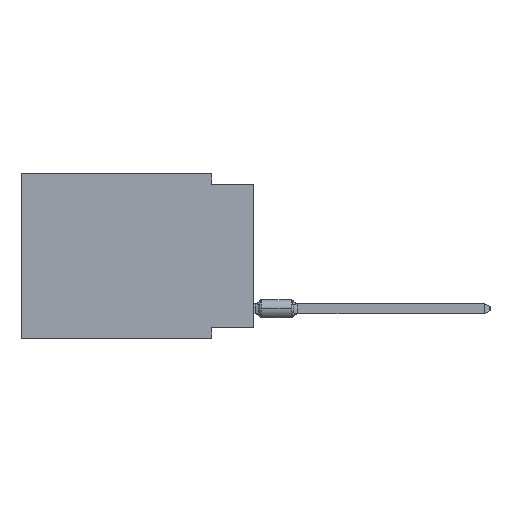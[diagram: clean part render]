
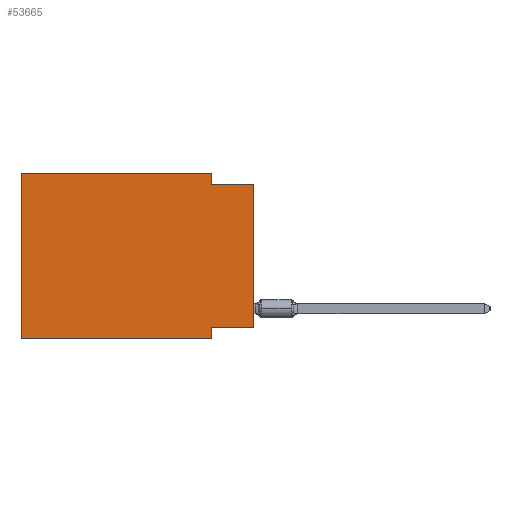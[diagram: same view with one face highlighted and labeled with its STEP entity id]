
A CAD part, left-side view. The second image highlights one B-rep face of the part: STEP entity #53665.
In plain terms, the highlighted planar face has unit normal (-1, 0, 0).
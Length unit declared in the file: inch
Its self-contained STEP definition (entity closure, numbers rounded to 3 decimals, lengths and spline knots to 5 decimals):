
#485 = LINE ( 'NONE', #64862, #18930 ) ;
#847 = VECTOR ( 'NONE', #35069, 39.37008 ) ;
#2722 = VERTEX_POINT ( 'NONE', #3172 ) ;
#2754 = EDGE_CURVE ( 'NONE', #50735, #27665, #9532, .T. ) ;
#3172 = CARTESIAN_POINT ( 'NONE',  ( 0., 0.1, -0.39 ) ) ;
#3854 = LINE ( 'NONE', #68250, #53950 ) ;
#4348 = ORIENTED_EDGE ( 'NONE', *, *, #4969, .F. ) ;
#4935 = CARTESIAN_POINT ( 'NONE',  ( 0., 0.55, -0.39 ) ) ;
#4969 = EDGE_CURVE ( 'NONE', #57707, #50735, #485, .T. ) ;
#5100 = VECTOR ( 'NONE', #33365, 39.37008 ) ;
#5515 = PLANE ( 'NONE',  #23063 ) ;
#7569 = DIRECTION ( 'NONE',  ( 0., -1., 0. ) ) ;
#9532 = LINE ( 'NONE', #15213, #26589 ) ;
#12675 = LINE ( 'NONE', #34378, #847 ) ;
#13250 = LINE ( 'NONE', #18584, #17897 ) ;
#13808 = EDGE_CURVE ( 'NONE', #33954, #2722, #12675, .T. ) ;
#15095 = ORIENTED_EDGE ( 'NONE', *, *, #56157, .F. ) ;
#15213 = CARTESIAN_POINT ( 'NONE',  ( 0., 0., -0.025 ) ) ;
#17350 = CARTESIAN_POINT ( 'NONE',  ( 0., 0.55, 0. ) ) ;
#17897 = VECTOR ( 'NONE', #7569, 39.37008 ) ;
#18584 = CARTESIAN_POINT ( 'NONE',  ( 0., 0.55, -0.39 ) ) ;
#18930 = VECTOR ( 'NONE', #43852, 39.37008 ) ;
#21472 = VECTOR ( 'NONE', #42526, 39.37008 ) ;
#21487 = DIRECTION ( 'NONE',  ( 1., 0., 0. ) ) ;
#21512 = CARTESIAN_POINT ( 'NONE',  ( 0., 0., 0. ) ) ;
#22717 = ORIENTED_EDGE ( 'NONE', *, *, #13808, .F. ) ;
#23063 = AXIS2_PLACEMENT_3D ( 'NONE', #27200, #21487, #48557 ) ;
#23834 = CARTESIAN_POINT ( 'NONE',  ( 0., 0., -0.025 ) ) ;
#24667 = LINE ( 'NONE', #51038, #26657 ) ;
#26589 = VECTOR ( 'NONE', #35866, 39.37008 ) ;
#26606 = LINE ( 'NONE', #17350, #5100 ) ;
#26657 = VECTOR ( 'NONE', #56712, 39.37008 ) ;
#26695 = EDGE_CURVE ( 'NONE', #30309, #27676, #26606, .T. ) ;
#27200 = CARTESIAN_POINT ( 'NONE',  ( 0., 0.55, 0. ) ) ;
#27665 = VERTEX_POINT ( 'NONE', #23834 ) ;
#27676 = VERTEX_POINT ( 'NONE', #45545 ) ;
#29125 = CARTESIAN_POINT ( 'NONE',  ( 0., 0.1, 0. ) ) ;
#29144 = VERTEX_POINT ( 'NONE', #60074 ) ;
#29556 = ORIENTED_EDGE ( 'NONE', *, *, #55874, .F. ) ;
#30309 = VERTEX_POINT ( 'NONE', #4935 ) ;
#31439 = EDGE_CURVE ( 'NONE', #30309, #2722, #13250, .T. ) ;
#33365 = DIRECTION ( 'NONE',  ( 0., 0., 1. ) ) ;
#33604 = CARTESIAN_POINT ( 'NONE',  ( 0., 0.1, -0.365 ) ) ;
#33954 = VERTEX_POINT ( 'NONE', #33604 ) ;
#34378 = CARTESIAN_POINT ( 'NONE',  ( 0., 0.1, -0.39 ) ) ;
#35069 = DIRECTION ( 'NONE',  ( 0., 0., -1. ) ) ;
#35866 = DIRECTION ( 'NONE',  ( 0., -1., 0. ) ) ;
#37516 = ORIENTED_EDGE ( 'NONE', *, *, #2754, .F. ) ;
#42526 = DIRECTION ( 'NONE',  ( 0., 0., 1. ) ) ;
#43382 = EDGE_LOOP ( 'NONE', ( #61867, #37516, #4348, #29556, #67159, #66904, #22717, #15095 ) ) ;
#43852 = DIRECTION ( 'NONE',  ( 0., 0., -1. ) ) ;
#45545 = CARTESIAN_POINT ( 'NONE',  ( 0., 0.55, 0. ) ) ;
#48557 = DIRECTION ( 'NONE',  ( 0., 0., -1. ) ) ;
#50735 = VERTEX_POINT ( 'NONE', #63160 ) ;
#51038 = CARTESIAN_POINT ( 'NONE',  ( 0., 0., -0.365 ) ) ;
#53665 = ADVANCED_FACE ( 'NONE', ( #65604 ), #5515, .F. ) ;
#53950 = VECTOR ( 'NONE', #62568, 39.37008 ) ;
#55874 = EDGE_CURVE ( 'NONE', #27676, #57707, #3854, .T. ) ;
#56157 = EDGE_CURVE ( 'NONE', #29144, #33954, #24667, .T. ) ;
#56712 = DIRECTION ( 'NONE',  ( 0., 1., 0. ) ) ;
#57707 = VERTEX_POINT ( 'NONE', #29125 ) ;
#58527 = LINE ( 'NONE', #21512, #21472 ) ;
#60074 = CARTESIAN_POINT ( 'NONE',  ( 0., 0., -0.365 ) ) ;
#61867 = ORIENTED_EDGE ( 'NONE', *, *, #68653, .T. ) ;
#62568 = DIRECTION ( 'NONE',  ( 0., -1., 0. ) ) ;
#63160 = CARTESIAN_POINT ( 'NONE',  ( 0., 0.1, -0.025 ) ) ;
#64862 = CARTESIAN_POINT ( 'NONE',  ( 0., 0.1, 0. ) ) ;
#65604 = FACE_OUTER_BOUND ( 'NONE', #43382, .T. ) ;
#66904 = ORIENTED_EDGE ( 'NONE', *, *, #31439, .T. ) ;
#67159 = ORIENTED_EDGE ( 'NONE', *, *, #26695, .F. ) ;
#68250 = CARTESIAN_POINT ( 'NONE',  ( 0., 0.55, 0. ) ) ;
#68653 = EDGE_CURVE ( 'NONE', #29144, #27665, #58527, .T. ) ;
